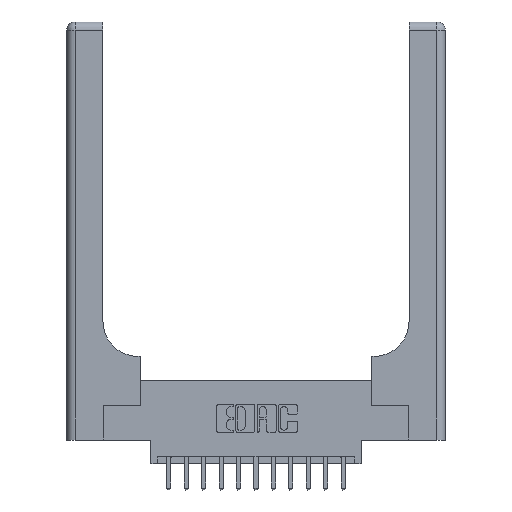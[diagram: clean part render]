
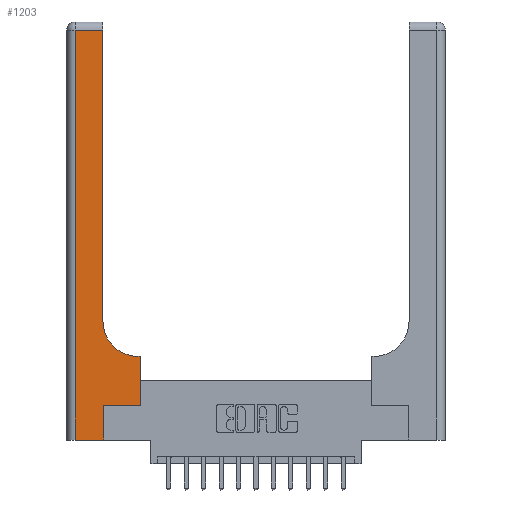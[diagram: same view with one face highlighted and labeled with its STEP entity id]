
A CAD part, top view. The second image highlights one B-rep face of the part: STEP entity #1203.
In plain terms, the highlighted planar face has unit normal (0, 0, 1).
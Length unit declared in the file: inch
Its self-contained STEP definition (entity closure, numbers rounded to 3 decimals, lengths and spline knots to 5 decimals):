
#307 = EDGE_CURVE ( 'NONE', #13820, #12424, #1714, .T. ) ;
#421 = CARTESIAN_POINT ( 'NONE',  ( 0.06, 3., 0.37 ) ) ;
#904 = DIRECTION ( 'NONE',  ( 0., 0., -1. ) ) ;
#1046 = VERTEX_POINT ( 'NONE', #12767 ) ;
#1158 = CARTESIAN_POINT ( 'NONE',  ( 0.265, 0.25, 0.37 ) ) ;
#1203 = ADVANCED_FACE ( 'NONE', ( #10202 ), #8538, .F. ) ;
#1298 = CARTESIAN_POINT ( 'NONE',  ( 0.26, 2.94, 0.37 ) ) ;
#1621 = CARTESIAN_POINT ( 'NONE',  ( 0.265, 0.25, 0.37 ) ) ;
#1695 = VECTOR ( 'NONE', #8710, 39.37008 ) ;
#1714 = LINE ( 'NONE', #8714, #1695 ) ;
#2452 = CARTESIAN_POINT ( 'NONE',  ( 0.26, 0.85, 0.37 ) ) ;
#2545 = ORIENTED_EDGE ( 'NONE', *, *, #6315, .T. ) ;
#2847 = VECTOR ( 'NONE', #10843, 39.37008 ) ;
#2954 = VERTEX_POINT ( 'NONE', #2452 ) ;
#2971 = ORIENTED_EDGE ( 'NONE', *, *, #6871, .T. ) ;
#3048 = VERTEX_POINT ( 'NONE', #1298 ) ;
#3268 = EDGE_CURVE ( 'NONE', #3048, #6038, #10547, .T. ) ;
#4140 = VERTEX_POINT ( 'NONE', #9390 ) ;
#4649 = VECTOR ( 'NONE', #7343, 39.37008 ) ;
#4940 = EDGE_CURVE ( 'NONE', #6038, #10513, #9886, .T. ) ;
#5428 = DIRECTION ( 'NONE',  ( -1., 0., 0. ) ) ;
#5474 = LINE ( 'NONE', #13158, #9273 ) ;
#5498 = DIRECTION ( 'NONE',  ( 0., 1., 0. ) ) ;
#5592 = EDGE_CURVE ( 'NONE', #15568, #4140, #8067, .T. ) ;
#6038 = VERTEX_POINT ( 'NONE', #16455 ) ;
#6315 = EDGE_CURVE ( 'NONE', #2954, #3048, #15510, .T. ) ;
#6593 = CIRCLE ( 'NONE', #7021, 0.25 ) ;
#6639 = VECTOR ( 'NONE', #14705, 39.37008 ) ;
#6871 = EDGE_CURVE ( 'NONE', #12424, #15568, #14327, .T. ) ;
#7021 = AXIS2_PLACEMENT_3D ( 'NONE', #8715, #904, #10007 ) ;
#7295 = ORIENTED_EDGE ( 'NONE', *, *, #307, .T. ) ;
#7343 = DIRECTION ( 'NONE',  ( 0., 1., 0. ) ) ;
#7618 = AXIS2_PLACEMENT_3D ( 'NONE', #8421, #8469, #8441 ) ;
#7935 = LINE ( 'NONE', #14460, #11367 ) ;
#8067 = LINE ( 'NONE', #15093, #4649 ) ;
#8421 = CARTESIAN_POINT ( 'NONE',  ( 0., 3., 0.37 ) ) ;
#8441 = DIRECTION ( 'NONE',  ( -1., 0., 0. ) ) ;
#8469 = DIRECTION ( 'NONE',  ( 0., 0., -1. ) ) ;
#8538 = PLANE ( 'NONE',  #7618 ) ;
#8557 = CARTESIAN_POINT ( 'NONE',  ( 0.265, 0., 0.37 ) ) ;
#8710 = DIRECTION ( 'NONE',  ( 0., 1., 0. ) ) ;
#8714 = CARTESIAN_POINT ( 'NONE',  ( 0.265, 0., 0.37 ) ) ;
#8715 = CARTESIAN_POINT ( 'NONE',  ( 0.51, 0.85, 0.37 ) ) ;
#9053 = ORIENTED_EDGE ( 'NONE', *, *, #4940, .T. ) ;
#9196 = ORIENTED_EDGE ( 'NONE', *, *, #11255, .T. ) ;
#9273 = VECTOR ( 'NONE', #5428, 39.37008 ) ;
#9390 = CARTESIAN_POINT ( 'NONE',  ( 0.528, 0.6, 0.37 ) ) ;
#9394 = ORIENTED_EDGE ( 'NONE', *, *, #3268, .T. ) ;
#9886 = LINE ( 'NONE', #421, #16319 ) ;
#10007 = DIRECTION ( 'NONE',  ( 1., 0., 0. ) ) ;
#10202 = FACE_OUTER_BOUND ( 'NONE', #15284, .T. ) ;
#10513 = VERTEX_POINT ( 'NONE', #13996 ) ;
#10547 = LINE ( 'NONE', #10734, #2847 ) ;
#10734 = CARTESIAN_POINT ( 'NONE',  ( 0., 2.94, 0.37 ) ) ;
#10843 = DIRECTION ( 'NONE',  ( -1., 0., 0. ) ) ;
#11255 = EDGE_CURVE ( 'NONE', #10513, #13820, #7935, .T. ) ;
#11367 = VECTOR ( 'NONE', #15729, 39.37008 ) ;
#12424 = VERTEX_POINT ( 'NONE', #1158 ) ;
#12767 = CARTESIAN_POINT ( 'NONE',  ( 0.51, 0.6, 0.37 ) ) ;
#13158 = CARTESIAN_POINT ( 'NONE',  ( 0.26, 0.6, 0.37 ) ) ;
#13328 = ORIENTED_EDGE ( 'NONE', *, *, #16705, .T. ) ;
#13474 = EDGE_CURVE ( 'NONE', #4140, #1046, #5474, .T. ) ;
#13820 = VERTEX_POINT ( 'NONE', #8557 ) ;
#13883 = ORIENTED_EDGE ( 'NONE', *, *, #13474, .T. ) ;
#13996 = CARTESIAN_POINT ( 'NONE',  ( 0.06, 0., 0.37 ) ) ;
#14167 = ORIENTED_EDGE ( 'NONE', *, *, #5592, .T. ) ;
#14296 = CARTESIAN_POINT ( 'NONE',  ( 0.528, 0.25, 0.37 ) ) ;
#14327 = LINE ( 'NONE', #1621, #6639 ) ;
#14460 = CARTESIAN_POINT ( 'NONE',  ( 0., 0., 0.37 ) ) ;
#14513 = CARTESIAN_POINT ( 'NONE',  ( 0.26, 3., 0.37 ) ) ;
#14705 = DIRECTION ( 'NONE',  ( 1., 0., 0. ) ) ;
#15093 = CARTESIAN_POINT ( 'NONE',  ( 0.528, 0.25, 0.37 ) ) ;
#15284 = EDGE_LOOP ( 'NONE', ( #2545, #9394, #9053, #9196, #7295, #2971, #14167, #13883, #13328 ) ) ;
#15510 = LINE ( 'NONE', #14513, #15915 ) ;
#15568 = VERTEX_POINT ( 'NONE', #14296 ) ;
#15729 = DIRECTION ( 'NONE',  ( 1., 0., 0. ) ) ;
#15915 = VECTOR ( 'NONE', #5498, 39.37008 ) ;
#16000 = DIRECTION ( 'NONE',  ( 0., -1., 0. ) ) ;
#16319 = VECTOR ( 'NONE', #16000, 39.37008 ) ;
#16455 = CARTESIAN_POINT ( 'NONE',  ( 0.06, 2.94, 0.37 ) ) ;
#16705 = EDGE_CURVE ( 'NONE', #1046, #2954, #6593, .T. ) ;
